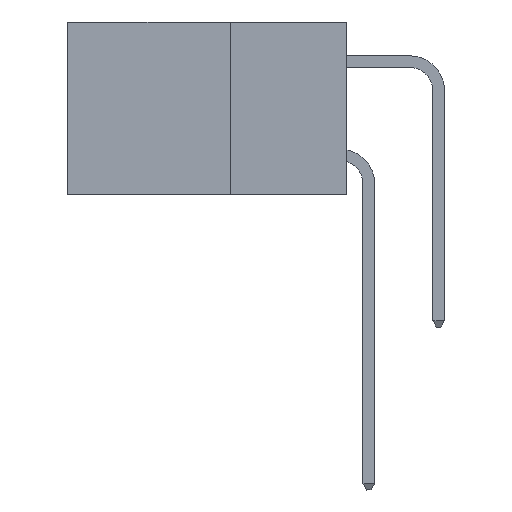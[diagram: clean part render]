
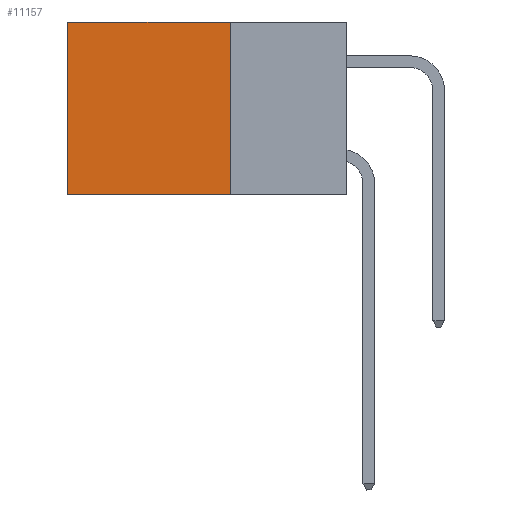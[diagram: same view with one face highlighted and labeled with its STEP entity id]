
A CAD part, left-side view. The second image highlights one B-rep face of the part: STEP entity #11157.
In plain terms, the highlighted planar face has unit normal (-1, 0, 0).
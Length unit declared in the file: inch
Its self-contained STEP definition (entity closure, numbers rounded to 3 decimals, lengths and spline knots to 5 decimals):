
#923 = LINE ( 'NONE', #2137, #9253 ) ;
#1208 = DIRECTION ( 'NONE',  ( 1., 0., 0. ) ) ;
#1406 = CARTESIAN_POINT ( 'NONE',  ( 0.2875, 0.25, 0. ) ) ;
#1568 = CARTESIAN_POINT ( 'NONE',  ( 0.2875, 0.25, 0. ) ) ;
#2137 = CARTESIAN_POINT ( 'NONE',  ( 0.2875, 0.25, 0. ) ) ;
#2251 = LINE ( 'NONE', #1406, #4677 ) ;
#2964 = FACE_OUTER_BOUND ( 'NONE', #9983, .T. ) ;
#3516 = DIRECTION ( 'NONE',  ( 0., 0., -1. ) ) ;
#3786 = CARTESIAN_POINT ( 'NONE',  ( 0.2875, 0.25, -0.37 ) ) ;
#4029 = ORIENTED_EDGE ( 'NONE', *, *, #6238, .F. ) ;
#4677 = VECTOR ( 'NONE', #3516, 39.37008 ) ;
#5887 = DIRECTION ( 'NONE',  ( 0., 0., -1. ) ) ;
#5912 = CARTESIAN_POINT ( 'NONE',  ( 0.2875, 0.6, -0.37 ) ) ;
#6238 = EDGE_CURVE ( 'NONE', #28603, #22137, #2251, .T. ) ;
#7607 = VERTEX_POINT ( 'NONE', #19544 ) ;
#7722 = ORIENTED_EDGE ( 'NONE', *, *, #15868, .F. ) ;
#9253 = VECTOR ( 'NONE', #10994, 39.37008 ) ;
#9983 = EDGE_LOOP ( 'NONE', ( #16410, #7722, #4029, #16791 ) ) ;
#10994 = DIRECTION ( 'NONE',  ( 0., 1., 0. ) ) ;
#11157 = ADVANCED_FACE ( 'NONE', ( #2964 ), #14339, .F. ) ;
#11294 = CARTESIAN_POINT ( 'NONE',  ( 0.2875, 0.25, -0.37 ) ) ;
#11305 = LINE ( 'NONE', #23518, #27961 ) ;
#14339 = PLANE ( 'NONE',  #28207 ) ;
#15868 = EDGE_CURVE ( 'NONE', #22137, #18787, #25592, .T. ) ;
#16410 = ORIENTED_EDGE ( 'NONE', *, *, #20368, .T. ) ;
#16791 = ORIENTED_EDGE ( 'NONE', *, *, #19989, .T. ) ;
#18787 = VERTEX_POINT ( 'NONE', #5912 ) ;
#19437 = DIRECTION ( 'NONE',  ( 0., 1., 0. ) ) ;
#19544 = CARTESIAN_POINT ( 'NONE',  ( 0.2875, 0.6, 0. ) ) ;
#19989 = EDGE_CURVE ( 'NONE', #28603, #7607, #923, .T. ) ;
#20368 = EDGE_CURVE ( 'NONE', #7607, #18787, #11305, .T. ) ;
#22137 = VERTEX_POINT ( 'NONE', #11294 ) ;
#22479 = VECTOR ( 'NONE', #19437, 39.37008 ) ;
#23518 = CARTESIAN_POINT ( 'NONE',  ( 0.2875, 0.6, 0. ) ) ;
#24591 = CARTESIAN_POINT ( 'NONE',  ( 0.2875, 0.25, 0. ) ) ;
#25592 = LINE ( 'NONE', #3786, #22479 ) ;
#27961 = VECTOR ( 'NONE', #5887, 39.37008 ) ;
#27972 = DIRECTION ( 'NONE',  ( 0., 0., -1. ) ) ;
#28207 = AXIS2_PLACEMENT_3D ( 'NONE', #1568, #1208, #27972 ) ;
#28603 = VERTEX_POINT ( 'NONE', #24591 ) ;
